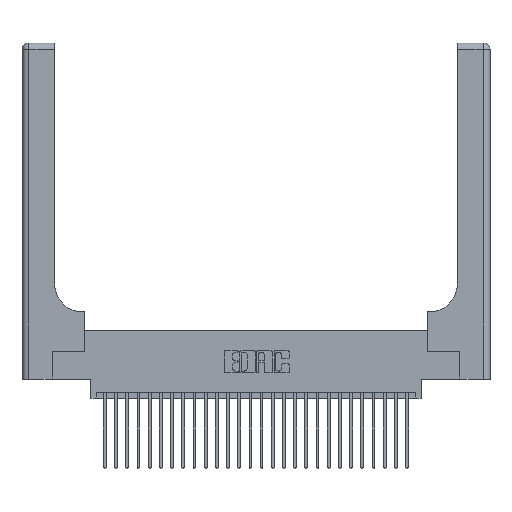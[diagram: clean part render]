
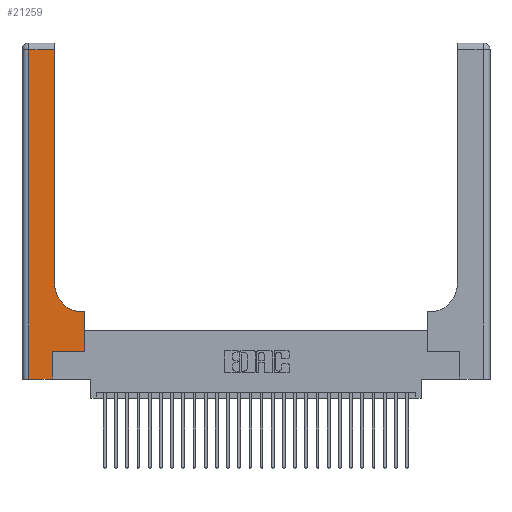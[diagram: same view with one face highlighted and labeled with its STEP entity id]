
A CAD part, top view. The second image highlights one B-rep face of the part: STEP entity #21259.
In plain terms, the highlighted planar face has unit normal (0, 0, 1).
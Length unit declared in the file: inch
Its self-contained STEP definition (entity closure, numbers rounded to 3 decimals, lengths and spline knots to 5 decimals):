
#194 = LINE ( 'NONE', #28713, #7630 ) ;
#526 = CARTESIAN_POINT ( 'NONE',  ( 0.2915, 3., 0.37 ) ) ;
#1267 = CIRCLE ( 'NONE', #11406, 0.25 ) ;
#1294 = CARTESIAN_POINT ( 'NONE',  ( 0.5415, 0.6, 0.37 ) ) ;
#1374 = CARTESIAN_POINT ( 'NONE',  ( 0.5585, 0.25, 0.37 ) ) ;
#2307 = DIRECTION ( 'NONE',  ( 0., 0., -1. ) ) ;
#2384 = CARTESIAN_POINT ( 'NONE',  ( 0.269, 0.25, 0.37 ) ) ;
#2409 = CARTESIAN_POINT ( 'NONE',  ( 0.06, 3., 0.37 ) ) ;
#2469 = EDGE_CURVE ( 'NONE', #5048, #17352, #26503, .T. ) ;
#2568 = VERTEX_POINT ( 'NONE', #4061 ) ;
#2761 = ORIENTED_EDGE ( 'NONE', *, *, #16323, .T. ) ;
#3091 = CARTESIAN_POINT ( 'NONE',  ( 0.2915, 0.85, 0.37 ) ) ;
#3233 = LINE ( 'NONE', #526, #14580 ) ;
#3929 = VECTOR ( 'NONE', #29046, 39.37008 ) ;
#4061 = CARTESIAN_POINT ( 'NONE',  ( 0.06, 0., 0.37 ) ) ;
#4668 = DIRECTION ( 'NONE',  ( 0., -1., 0. ) ) ;
#4717 = VECTOR ( 'NONE', #26102, 39.37008 ) ;
#5048 = VERTEX_POINT ( 'NONE', #1374 ) ;
#5956 = CARTESIAN_POINT ( 'NONE',  ( 0.5585, 0.25, 0.37 ) ) ;
#6593 = VERTEX_POINT ( 'NONE', #27028 ) ;
#7292 = CARTESIAN_POINT ( 'NONE',  ( 0.5585, 0.6, 0.37 ) ) ;
#7480 = ORIENTED_EDGE ( 'NONE', *, *, #19728, .T. ) ;
#7611 = VECTOR ( 'NONE', #12201, 39.37008 ) ;
#7630 = VECTOR ( 'NONE', #17577, 39.37008 ) ;
#7692 = VECTOR ( 'NONE', #4668, 39.37008 ) ;
#7716 = ORIENTED_EDGE ( 'NONE', *, *, #19736, .T. ) ;
#8288 = ORIENTED_EDGE ( 'NONE', *, *, #2469, .T. ) ;
#9220 = LINE ( 'NONE', #13334, #3929 ) ;
#9844 = EDGE_CURVE ( 'NONE', #21492, #28977, #3233, .T. ) ;
#10255 = CARTESIAN_POINT ( 'NONE',  ( 0.2915, 2.94, 0.37 ) ) ;
#11037 = CARTESIAN_POINT ( 'NONE',  ( 0., 0., 0.37 ) ) ;
#11406 = AXIS2_PLACEMENT_3D ( 'NONE', #25105, #11558, #27317 ) ;
#11558 = DIRECTION ( 'NONE',  ( 0., 0., -1. ) ) ;
#11770 = DIRECTION ( 'NONE',  ( 0., 1., 0. ) ) ;
#12201 = DIRECTION ( 'NONE',  ( 1., 0., 0. ) ) ;
#13334 = CARTESIAN_POINT ( 'NONE',  ( 0.269, 0., 0.37 ) ) ;
#13634 = LINE ( 'NONE', #21232, #7611 ) ;
#13785 = FACE_OUTER_BOUND ( 'NONE', #25405, .T. ) ;
#13990 = ORIENTED_EDGE ( 'NONE', *, *, #16585, .T. ) ;
#14580 = VECTOR ( 'NONE', #11770, 39.37008 ) ;
#15684 = ORIENTED_EDGE ( 'NONE', *, *, #9844, .T. ) ;
#15892 = CARTESIAN_POINT ( 'NONE',  ( 0., 3., 0.37 ) ) ;
#16323 = EDGE_CURVE ( 'NONE', #28977, #6593, #194, .T. ) ;
#16585 = EDGE_CURVE ( 'NONE', #19533, #21492, #1267, .T. ) ;
#17195 = CARTESIAN_POINT ( 'NONE',  ( 0.2915, 0.6, 0.37 ) ) ;
#17352 = VERTEX_POINT ( 'NONE', #7292 ) ;
#17451 = EDGE_CURVE ( 'NONE', #25464, #5048, #13634, .T. ) ;
#17577 = DIRECTION ( 'NONE',  ( -1., 0., 0. ) ) ;
#18178 = DIRECTION ( 'NONE',  ( -1., 0., 0. ) ) ;
#19121 = ORIENTED_EDGE ( 'NONE', *, *, #24666, .T. ) ;
#19533 = VERTEX_POINT ( 'NONE', #1294 ) ;
#19544 = DIRECTION ( 'NONE',  ( 0., 1., 0. ) ) ;
#19728 = EDGE_CURVE ( 'NONE', #25284, #25464, #9220, .T. ) ;
#19736 = EDGE_CURVE ( 'NONE', #2568, #25284, #21271, .T. ) ;
#19871 = VECTOR ( 'NONE', #19544, 39.37008 ) ;
#21232 = CARTESIAN_POINT ( 'NONE',  ( 0.269, 0.25, 0.37 ) ) ;
#21259 = ADVANCED_FACE ( 'NONE', ( #13785 ), #22579, .F. ) ;
#21271 = LINE ( 'NONE', #11037, #26515 ) ;
#21492 = VERTEX_POINT ( 'NONE', #3091 ) ;
#22579 = PLANE ( 'NONE',  #28852 ) ;
#24226 = CARTESIAN_POINT ( 'NONE',  ( 0.269, 0., 0.37 ) ) ;
#24579 = DIRECTION ( 'NONE',  ( 1., 0., 0. ) ) ;
#24666 = EDGE_CURVE ( 'NONE', #17352, #19533, #28695, .T. ) ;
#25004 = LINE ( 'NONE', #2409, #7692 ) ;
#25105 = CARTESIAN_POINT ( 'NONE',  ( 0.5415, 0.85, 0.37 ) ) ;
#25284 = VERTEX_POINT ( 'NONE', #24226 ) ;
#25405 = EDGE_LOOP ( 'NONE', ( #15684, #2761, #27168, #7716, #7480, #26132, #8288, #19121, #13990 ) ) ;
#25464 = VERTEX_POINT ( 'NONE', #2384 ) ;
#26102 = DIRECTION ( 'NONE',  ( -1., 0., 0. ) ) ;
#26132 = ORIENTED_EDGE ( 'NONE', *, *, #17451, .T. ) ;
#26503 = LINE ( 'NONE', #5956, #19871 ) ;
#26515 = VECTOR ( 'NONE', #24579, 39.37008 ) ;
#27028 = CARTESIAN_POINT ( 'NONE',  ( 0.06, 2.94, 0.37 ) ) ;
#27168 = ORIENTED_EDGE ( 'NONE', *, *, #27984, .T. ) ;
#27317 = DIRECTION ( 'NONE',  ( 1., 0., 0. ) ) ;
#27984 = EDGE_CURVE ( 'NONE', #6593, #2568, #25004, .T. ) ;
#28695 = LINE ( 'NONE', #17195, #4717 ) ;
#28713 = CARTESIAN_POINT ( 'NONE',  ( 0., 2.94, 0.37 ) ) ;
#28852 = AXIS2_PLACEMENT_3D ( 'NONE', #15892, #2307, #18178 ) ;
#28977 = VERTEX_POINT ( 'NONE', #10255 ) ;
#29046 = DIRECTION ( 'NONE',  ( 0., 1., 0. ) ) ;
